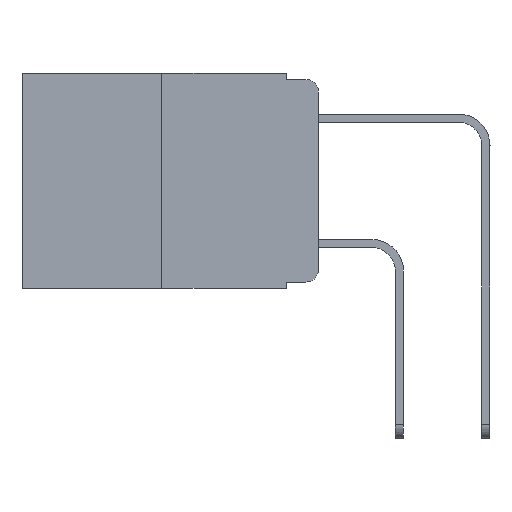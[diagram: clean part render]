
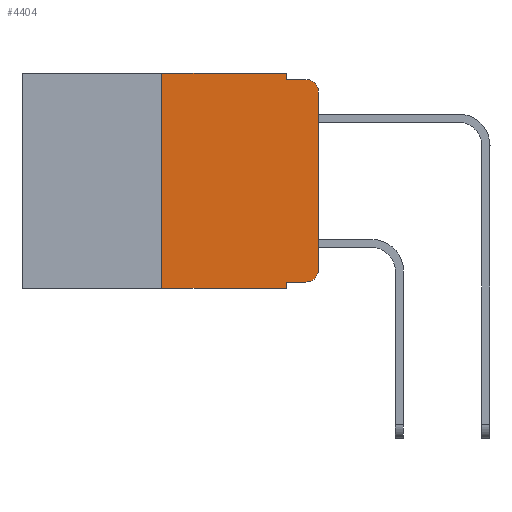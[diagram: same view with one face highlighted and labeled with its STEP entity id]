
A CAD part, left-side view. The second image highlights one B-rep face of the part: STEP entity #4404.
In plain terms, the highlighted planar face has unit normal (-1, 0, 0).
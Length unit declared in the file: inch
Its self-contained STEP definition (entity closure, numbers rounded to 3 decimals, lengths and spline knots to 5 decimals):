
#104 = DIRECTION ( 'NONE',  ( 0., -1., 0. ) ) ;
#175 = AXIS2_PLACEMENT_3D ( 'NONE', #10743, #14473, #3573 ) ;
#457 = ORIENTED_EDGE ( 'NONE', *, *, #7525, .F. ) ;
#589 = FACE_OUTER_BOUND ( 'NONE', #8068, .T. ) ;
#643 = VECTOR ( 'NONE', #6249, 39.37008 ) ;
#952 = CARTESIAN_POINT ( 'NONE',  ( 0., 0.051, -0.01 ) ) ;
#1055 = VERTEX_POINT ( 'NONE', #952 ) ;
#1244 = VERTEX_POINT ( 'NONE', #1293 ) ;
#1293 = CARTESIAN_POINT ( 'NONE',  ( 0., 0.02, -0.01 ) ) ;
#1342 = EDGE_CURVE ( 'NONE', #8441, #10855, #1586, .T. ) ;
#1430 = EDGE_CURVE ( 'NONE', #14414, #3388, #13922, .T. ) ;
#1524 = DIRECTION ( 'NONE',  ( 0., 0., -1. ) ) ;
#1586 = LINE ( 'NONE', #14348, #7909 ) ;
#1966 = CIRCLE ( 'NONE', #175, 0.02 ) ;
#2095 = ORIENTED_EDGE ( 'NONE', *, *, #1342, .T. ) ;
#2188 = VECTOR ( 'NONE', #14336, 39.37008 ) ;
#2349 = AXIS2_PLACEMENT_3D ( 'NONE', #9571, #5877, #13285 ) ;
#2878 = EDGE_CURVE ( 'NONE', #8441, #4835, #7474, .T. ) ;
#3181 = EDGE_CURVE ( 'NONE', #10855, #14414, #8979, .T. ) ;
#3388 = VERTEX_POINT ( 'NONE', #6849 ) ;
#3430 = ORIENTED_EDGE ( 'NONE', *, *, #15345, .T. ) ;
#3436 = CARTESIAN_POINT ( 'NONE',  ( 0., 0., 0. ) ) ;
#3573 = DIRECTION ( 'NONE',  ( 0., 0., -1. ) ) ;
#3734 = CARTESIAN_POINT ( 'NONE',  ( 0., 0.473, -0.343 ) ) ;
#4404 = ADVANCED_FACE ( 'NONE', ( #589 ), #13060, .F. ) ;
#4550 = CARTESIAN_POINT ( 'NONE',  ( 0., 0.25, -0.343 ) ) ;
#4565 = LINE ( 'NONE', #10614, #2188 ) ;
#4656 = ORIENTED_EDGE ( 'NONE', *, *, #7010, .T. ) ;
#4664 = VECTOR ( 'NONE', #15336, 39.37008 ) ;
#4835 = VERTEX_POINT ( 'NONE', #5399 ) ;
#5399 = CARTESIAN_POINT ( 'NONE',  ( 0., 0.051, -0.343 ) ) ;
#5707 = CARTESIAN_POINT ( 'NONE',  ( 0., 0.25, 0. ) ) ;
#5864 = DIRECTION ( 'NONE',  ( 0., -1., 0. ) ) ;
#5877 = DIRECTION ( 'NONE',  ( 1., 0., 0. ) ) ;
#5913 = VERTEX_POINT ( 'NONE', #11159 ) ;
#6249 = DIRECTION ( 'NONE',  ( 0., -1., 0. ) ) ;
#6424 = CARTESIAN_POINT ( 'NONE',  ( 0., 0.051, -0.333 ) ) ;
#6849 = CARTESIAN_POINT ( 'NONE',  ( 0., 0., -0.03 ) ) ;
#6983 = ORIENTED_EDGE ( 'NONE', *, *, #1430, .T. ) ;
#7010 = EDGE_CURVE ( 'NONE', #7437, #4835, #15020, .T. ) ;
#7437 = VERTEX_POINT ( 'NONE', #4550 ) ;
#7474 = LINE ( 'NONE', #15482, #12916 ) ;
#7525 = EDGE_CURVE ( 'NONE', #7437, #15237, #12559, .T. ) ;
#7909 = VECTOR ( 'NONE', #104, 39.37008 ) ;
#8068 = EDGE_LOOP ( 'NONE', ( #6983, #3430, #8658, #12354, #9604, #457, #4656, #9468, #2095, #10451 ) ) ;
#8441 = VERTEX_POINT ( 'NONE', #6424 ) ;
#8565 = CARTESIAN_POINT ( 'NONE',  ( 0., 0.02, -0.313 ) ) ;
#8658 = ORIENTED_EDGE ( 'NONE', *, *, #10389, .F. ) ;
#8979 = CIRCLE ( 'NONE', #10527, 0.02 ) ;
#9055 = CARTESIAN_POINT ( 'NONE',  ( 0., 0., -0.313 ) ) ;
#9286 = VECTOR ( 'NONE', #5864, 39.37008 ) ;
#9320 = LINE ( 'NONE', #10655, #11741 ) ;
#9468 = ORIENTED_EDGE ( 'NONE', *, *, #2878, .F. ) ;
#9495 = CARTESIAN_POINT ( 'NONE',  ( 0., 0.02, -0.333 ) ) ;
#9571 = CARTESIAN_POINT ( 'NONE',  ( 0., 0.473, 0. ) ) ;
#9604 = ORIENTED_EDGE ( 'NONE', *, *, #14618, .F. ) ;
#10389 = EDGE_CURVE ( 'NONE', #1055, #1244, #10402, .T. ) ;
#10402 = LINE ( 'NONE', #11743, #9286 ) ;
#10451 = ORIENTED_EDGE ( 'NONE', *, *, #3181, .T. ) ;
#10527 = AXIS2_PLACEMENT_3D ( 'NONE', #8565, #13549, #1524 ) ;
#10614 = CARTESIAN_POINT ( 'NONE',  ( 0., 0.473, 0. ) ) ;
#10655 = CARTESIAN_POINT ( 'NONE',  ( 0., 0.051, 0. ) ) ;
#10719 = VECTOR ( 'NONE', #12854, 39.37008 ) ;
#10743 = CARTESIAN_POINT ( 'NONE',  ( 0., 0.02, -0.03 ) ) ;
#10855 = VERTEX_POINT ( 'NONE', #9495 ) ;
#11159 = CARTESIAN_POINT ( 'NONE',  ( 0., 0.051, 0. ) ) ;
#11741 = VECTOR ( 'NONE', #14274, 39.37008 ) ;
#11743 = CARTESIAN_POINT ( 'NONE',  ( 0., 0.051, -0.01 ) ) ;
#11854 = CARTESIAN_POINT ( 'NONE',  ( 0., 0.25, 0. ) ) ;
#12050 = DIRECTION ( 'NONE',  ( 0., 0., -1. ) ) ;
#12354 = ORIENTED_EDGE ( 'NONE', *, *, #14135, .F. ) ;
#12559 = LINE ( 'NONE', #11854, #4664 ) ;
#12854 = DIRECTION ( 'NONE',  ( 0., 0., 1. ) ) ;
#12916 = VECTOR ( 'NONE', #12050, 39.37008 ) ;
#13060 = PLANE ( 'NONE',  #2349 ) ;
#13285 = DIRECTION ( 'NONE',  ( 0., 0., -1. ) ) ;
#13549 = DIRECTION ( 'NONE',  ( -1., 0., 0. ) ) ;
#13922 = LINE ( 'NONE', #3436, #10719 ) ;
#14135 = EDGE_CURVE ( 'NONE', #5913, #1055, #9320, .T. ) ;
#14274 = DIRECTION ( 'NONE',  ( 0., 0., -1. ) ) ;
#14336 = DIRECTION ( 'NONE',  ( 0., -1., 0. ) ) ;
#14348 = CARTESIAN_POINT ( 'NONE',  ( 0., 0.051, -0.333 ) ) ;
#14414 = VERTEX_POINT ( 'NONE', #9055 ) ;
#14473 = DIRECTION ( 'NONE',  ( -1., 0., 0. ) ) ;
#14618 = EDGE_CURVE ( 'NONE', #15237, #5913, #4565, .T. ) ;
#15020 = LINE ( 'NONE', #3734, #643 ) ;
#15237 = VERTEX_POINT ( 'NONE', #5707 ) ;
#15336 = DIRECTION ( 'NONE',  ( 0., 0., 1. ) ) ;
#15345 = EDGE_CURVE ( 'NONE', #3388, #1244, #1966, .T. ) ;
#15482 = CARTESIAN_POINT ( 'NONE',  ( 0., 0.051, 0. ) ) ;
